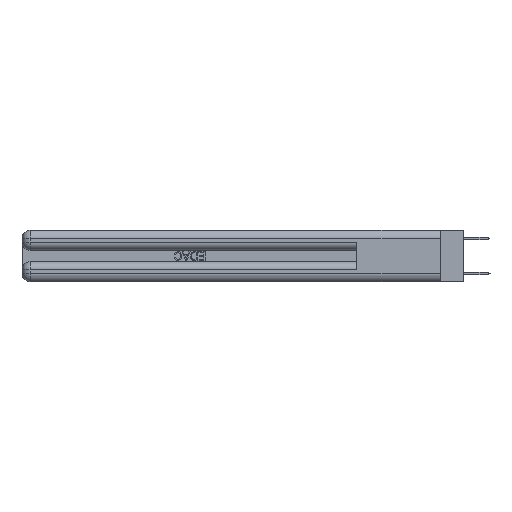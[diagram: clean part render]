
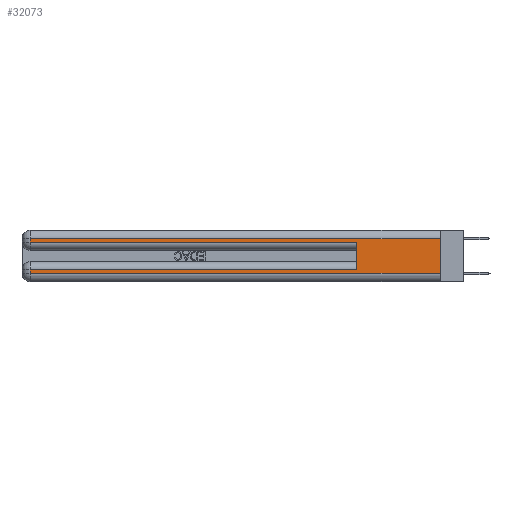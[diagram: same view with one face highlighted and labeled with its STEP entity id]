
A CAD part, left-side view. The second image highlights one B-rep face of the part: STEP entity #32073.
In plain terms, the highlighted planar face has unit normal (-1, 0, 0).
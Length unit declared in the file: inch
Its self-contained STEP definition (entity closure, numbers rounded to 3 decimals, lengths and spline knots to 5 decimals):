
#837 = ORIENTED_EDGE ( 'NONE', *, *, #22095, .F. ) ;
#1109 = DIRECTION ( 'NONE',  ( 0., 0., 1. ) ) ;
#1244 = VECTOR ( 'NONE', #1109, 39.37008 ) ;
#1614 = EDGE_CURVE ( 'NONE', #13287, #3524, #7829, .T. ) ;
#1672 = CARTESIAN_POINT ( 'NONE',  ( 0., 2.94, 0.085 ) ) ;
#1922 = CARTESIAN_POINT ( 'NONE',  ( 0., 0., 0.37 ) ) ;
#2922 = CARTESIAN_POINT ( 'NONE',  ( 0., 0., 0.285 ) ) ;
#3524 = VERTEX_POINT ( 'NONE', #6666 ) ;
#4482 = CARTESIAN_POINT ( 'NONE',  ( 0., 2.94, 0.31 ) ) ;
#5205 = DIRECTION ( 'NONE',  ( 0., 1., 0. ) ) ;
#5390 = LINE ( 'NONE', #17507, #19330 ) ;
#5498 = ORIENTED_EDGE ( 'NONE', *, *, #26344, .T. ) ;
#5922 = ORIENTED_EDGE ( 'NONE', *, *, #9819, .T. ) ;
#6413 = DIRECTION ( 'NONE',  ( 0., 0., -1. ) ) ;
#6499 = VECTOR ( 'NONE', #5205, 39.37008 ) ;
#6666 = CARTESIAN_POINT ( 'NONE',  ( 0., 0.6, 0.285 ) ) ;
#7533 = PLANE ( 'NONE',  #33965 ) ;
#7594 = ORIENTED_EDGE ( 'NONE', *, *, #27024, .T. ) ;
#7829 = LINE ( 'NONE', #15029, #1244 ) ;
#8923 = CARTESIAN_POINT ( 'NONE',  ( 0., 2.94, 0.285 ) ) ;
#9819 = EDGE_CURVE ( 'NONE', #13287, #24195, #13909, .T. ) ;
#10079 = CARTESIAN_POINT ( 'NONE',  ( 0., 0., 0.06 ) ) ;
#10228 = CARTESIAN_POINT ( 'NONE',  ( 0., 0., 0.31 ) ) ;
#10299 = VERTEX_POINT ( 'NONE', #34370 ) ;
#10364 = DIRECTION ( 'NONE',  ( 0., 0., -1. ) ) ;
#11516 = VERTEX_POINT ( 'NONE', #10228 ) ;
#12015 = LINE ( 'NONE', #27959, #25711 ) ;
#12161 = DIRECTION ( 'NONE',  ( 0., 0., -1. ) ) ;
#12763 = VERTEX_POINT ( 'NONE', #4482 ) ;
#12840 = EDGE_CURVE ( 'NONE', #11516, #12763, #15199, .T. ) ;
#13287 = VERTEX_POINT ( 'NONE', #25765 ) ;
#13909 = LINE ( 'NONE', #24372, #6499 ) ;
#14385 = ORIENTED_EDGE ( 'NONE', *, *, #12840, .T. ) ;
#14705 = EDGE_CURVE ( 'NONE', #12763, #18551, #24895, .T. ) ;
#15029 = CARTESIAN_POINT ( 'NONE',  ( 0., 0.6, 0.145 ) ) ;
#15199 = LINE ( 'NONE', #26849, #28735 ) ;
#15517 = ORIENTED_EDGE ( 'NONE', *, *, #19156, .T. ) ;
#17507 = CARTESIAN_POINT ( 'NONE',  ( 0., 2.94, 0.37 ) ) ;
#18158 = VECTOR ( 'NONE', #22408, 39.37008 ) ;
#18551 = VERTEX_POINT ( 'NONE', #8923 ) ;
#19156 = EDGE_CURVE ( 'NONE', #24195, #10299, #5390, .T. ) ;
#19330 = VECTOR ( 'NONE', #6413, 39.37008 ) ;
#19730 = DIRECTION ( 'NONE',  ( 0., 0., -1. ) ) ;
#20894 = ORIENTED_EDGE ( 'NONE', *, *, #1614, .F. ) ;
#22095 = EDGE_CURVE ( 'NONE', #11516, #30755, #30426, .T. ) ;
#22408 = DIRECTION ( 'NONE',  ( 0., -1., 0. ) ) ;
#23795 = ORIENTED_EDGE ( 'NONE', *, *, #14705, .T. ) ;
#24195 = VERTEX_POINT ( 'NONE', #1672 ) ;
#24372 = CARTESIAN_POINT ( 'NONE',  ( 0., 0., 0.085 ) ) ;
#24895 = LINE ( 'NONE', #33819, #31128 ) ;
#25349 = LINE ( 'NONE', #2922, #18158 ) ;
#25711 = VECTOR ( 'NONE', #30638, 39.37008 ) ;
#25765 = CARTESIAN_POINT ( 'NONE',  ( 0., 0.6, 0.085 ) ) ;
#26344 = EDGE_CURVE ( 'NONE', #18551, #3524, #25349, .T. ) ;
#26750 = DIRECTION ( 'NONE',  ( 1., 0., 0. ) ) ;
#26849 = CARTESIAN_POINT ( 'NONE',  ( 0., 0., 0.31 ) ) ;
#27024 = EDGE_CURVE ( 'NONE', #10299, #30755, #12015, .T. ) ;
#27796 = CARTESIAN_POINT ( 'NONE',  ( 0., 0., 0.37 ) ) ;
#27959 = CARTESIAN_POINT ( 'NONE',  ( 0., 0., 0.06 ) ) ;
#28077 = EDGE_LOOP ( 'NONE', ( #837, #14385, #23795, #5498, #20894, #5922, #15517, #7594 ) ) ;
#28735 = VECTOR ( 'NONE', #29490, 39.37008 ) ;
#29490 = DIRECTION ( 'NONE',  ( 0., 1., 0. ) ) ;
#29582 = VECTOR ( 'NONE', #19730, 39.37008 ) ;
#30426 = LINE ( 'NONE', #27796, #29582 ) ;
#30638 = DIRECTION ( 'NONE',  ( 0., -1., 0. ) ) ;
#30755 = VERTEX_POINT ( 'NONE', #10079 ) ;
#31128 = VECTOR ( 'NONE', #12161, 39.37008 ) ;
#32073 = ADVANCED_FACE ( 'NONE', ( #33192 ), #7533, .F. ) ;
#33192 = FACE_OUTER_BOUND ( 'NONE', #28077, .T. ) ;
#33819 = CARTESIAN_POINT ( 'NONE',  ( 0., 2.94, 0.37 ) ) ;
#33965 = AXIS2_PLACEMENT_3D ( 'NONE', #1922, #26750, #10364 ) ;
#34370 = CARTESIAN_POINT ( 'NONE',  ( 0., 2.94, 0.06 ) ) ;
